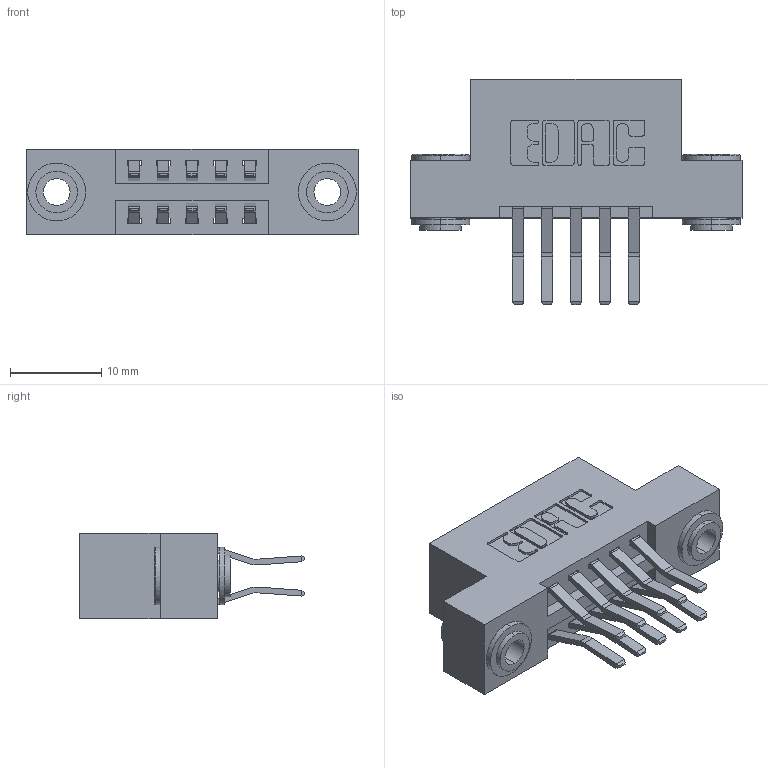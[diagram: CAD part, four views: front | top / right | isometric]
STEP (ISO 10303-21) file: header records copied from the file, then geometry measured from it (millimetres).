
FILE_DESCRIPTION (( 'STEP AP203' ), '1' );
FILE_NAME ('396-010-560-203.STEP', '2019-10-29T19:07:51', ( '' ), ( '' ), 'SwSTEP 2.0', 'SolidWorks 2016', '' );
FILE_SCHEMA (( 'CONFIG_CONTROL_DESIGN' ));
Length unit declared in the file: inch
Products named in the file (4): 345-250-002_345-250-002-102; 345-292-001_560 Tail; 346 Part_Flush Mounting Lugs - 0.156 Dia-TH; 396-010-560-203
Assembly tree (13 placements, depth 2):
  396-010-560-203
    346 Part_Flush Mounting Lugs - 0.156 Dia-TH
    345-292-001_560 Tail  x10
    345-250-002_345-250-002-102  x2
Bounding box: 36.45 x 24.78 x 9.4 mm (x, y, z)
Volume: 3351.8 mm3; surface area: 4414.8 mm2
Topology: 13 solids, 13 shells, 700 faces, 2015 edges, 1326 vertices
Faces by surface type: plane 436, cylinder 256, cone 8
Entity records: 8982 total; most frequent: CARTESIAN_POINT 1507, ORIENTED_EDGE 1434, DIRECTION 1415, EDGE_CURVE 717, LINE 537, VECTOR 537, VERTEX_POINT 474, AXIS2_PLACEMENT_3D 439
